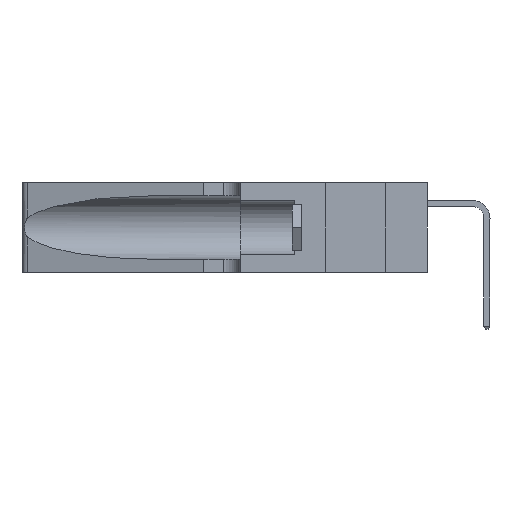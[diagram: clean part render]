
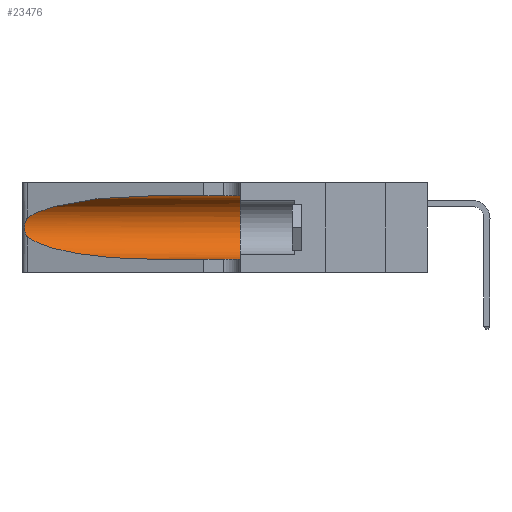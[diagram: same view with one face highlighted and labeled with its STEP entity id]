
A CAD part, left-side view. The second image highlights one B-rep face of the part: STEP entity #23476.
In plain terms, the highlighted cylindrical face has radius 3.308 mm (diameter 6.617 mm), a partial arc.
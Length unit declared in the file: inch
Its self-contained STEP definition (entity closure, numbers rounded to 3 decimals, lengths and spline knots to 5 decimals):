
#197 = VERTEX_POINT ( 'NONE', #7270 ) ;
#234 =( BOUNDED_CURVE ( )  B_SPLINE_CURVE ( 3, ( #10838, #6887, #12788, #996 ),
 .UNSPECIFIED., .F., .F. ) 
 B_SPLINE_CURVE_WITH_KNOTS ( ( 4, 4 ),
 ( 1.5708, 2.84003 ),
 .UNSPECIFIED. ) 
 CURVE ( )  GEOMETRIC_REPRESENTATION_ITEM ( )  RATIONAL_B_SPLINE_CURVE ( ( 1., 0.87, 0.87, 1. ) ) 
 REPRESENTATION_ITEM ( '' )  );
#996 = CARTESIAN_POINT ( 'NONE',  ( 0.25487, 1.22718, 0.22369 ) ) ;
#1383 = CARTESIAN_POINT ( 'NONE',  ( 0.1305, 0.72297, 0.05475 ) ) ;
#1867 = CARTESIAN_POINT ( 'NONE',  ( 0.25854, 1.2359, 0.20912 ) ) ;
#3170 = EDGE_CURVE ( 'NONE', #6573, #18868, #19099, .T. ) ;
#3399 = CARTESIAN_POINT ( 'NONE',  ( 0.1305, 0.35, 0.31525 ) ) ;
#3686 = VERTEX_POINT ( 'NONE', #19341 ) ;
#3841 = CARTESIAN_POINT ( 'NONE',  ( 0.26075, 1.23896, 0.19203 ) ) ;
#3850 = CARTESIAN_POINT ( 'NONE',  ( 0.1305, 1.61858, 0.05475 ) ) ;
#4931 = CIRCLE ( 'NONE', #16431, 0.13025 ) ;
#5679 = EDGE_CURVE ( 'NONE', #18096, #3686, #4931, .T. ) ;
#5727 = ORIENTED_EDGE ( 'NONE', *, *, #15641, .T. ) ;
#5842 = CARTESIAN_POINT ( 'NONE',  ( 0.26017, 1.23833, 0.17102 ) ) ;
#5984 = DIRECTION ( 'NONE',  ( 0., 0., -1. ) ) ;
#6308 = ORIENTED_EDGE ( 'NONE', *, *, #7146, .T. ) ;
#6573 = VERTEX_POINT ( 'NONE', #15564 ) ;
#6686 = AXIS2_PLACEMENT_3D ( 'NONE', #7915, #17740, #5984 ) ;
#6887 = CARTESIAN_POINT ( 'NONE',  ( 0.18966, 0.96281, 0.31525 ) ) ;
#7146 = EDGE_CURVE ( 'NONE', #9513, #6573, #13261, .T. ) ;
#7270 = CARTESIAN_POINT ( 'NONE',  ( 0.1305, 0.72297, 0.31525 ) ) ;
#7305 = ORIENTED_EDGE ( 'NONE', *, *, #3170, .T. ) ;
#7864 = CARTESIAN_POINT ( 'NONE',  ( 0.25789, 1.23486, 0.15765 ) ) ;
#7915 = CARTESIAN_POINT ( 'NONE',  ( 0.1305, 1.61858, 0.185 ) ) ;
#8028 = DIRECTION ( 'NONE',  ( 0., 1., 0. ) ) ;
#8555 = ORIENTED_EDGE ( 'NONE', *, *, #11719, .F. ) ;
#9513 = VERTEX_POINT ( 'NONE', #10595 ) ;
#9820 = CARTESIAN_POINT ( 'NONE',  ( 0.25555, 1.22993, 0.14849 ) ) ;
#10198 = CARTESIAN_POINT ( 'NONE',  ( 0.1305, 0.72297, 0.05475 ) ) ;
#10595 = CARTESIAN_POINT ( 'NONE',  ( 0.25487, 1.22718, 0.22369 ) ) ;
#10838 = CARTESIAN_POINT ( 'NONE',  ( 0.1305, 0.72297, 0.31525 ) ) ;
#11719 = EDGE_CURVE ( 'NONE', #197, #18096, #17333, .T. ) ;
#11855 = DIRECTION ( 'NONE',  ( 0., -1., 0. ) ) ;
#12130 = VECTOR ( 'NONE', #11855, 39.37008 ) ;
#12788 = CARTESIAN_POINT ( 'NONE',  ( 0.2373, 1.15595, 0.28018 ) ) ;
#13184 = CARTESIAN_POINT ( 'NONE',  ( 0.25487, 1.22718, 0.14631 ) ) ;
#13261 = B_SPLINE_CURVE_WITH_KNOTS ( 'NONE', 3,
 ( #23358, #21391, #25306, #13660, #1867, #15634, #3841, #17598, #5842, #19524, #7864, #21470, #9820, #23446 ),
 .UNSPECIFIED., .F., .F.,
 ( 4, 2, 2, 2, 2, 2, 4 ),
 ( 0., 0.00027, 0.00053, 0.00107, 0.0016, 0.00187, 0.00214 ),
 .UNSPECIFIED. ) ;
#13660 = CARTESIAN_POINT ( 'NONE',  ( 0.25787, 1.23484, 0.2124 ) ) ;
#13671 = DIRECTION ( 'NONE',  ( 0., -1., 0. ) ) ;
#13778 = LINE ( 'NONE', #3850, #18355 ) ;
#13823 = CARTESIAN_POINT ( 'NONE',  ( 0.1305, 1.61858, 0.31525 ) ) ;
#15351 = FACE_OUTER_BOUND ( 'NONE', #18845, .T. ) ;
#15564 = CARTESIAN_POINT ( 'NONE',  ( 0.25487, 1.22718, 0.14631 ) ) ;
#15634 = CARTESIAN_POINT ( 'NONE',  ( 0.26018, 1.23835, 0.19895 ) ) ;
#15641 = EDGE_CURVE ( 'NONE', #18868, #3686, #13778, .T. ) ;
#16431 = AXIS2_PLACEMENT_3D ( 'NONE', #19682, #8028, #21636 ) ;
#16506 = EDGE_CURVE ( 'NONE', #197, #9513, #234, .T. ) ;
#17333 = LINE ( 'NONE', #13823, #12130 ) ;
#17598 = CARTESIAN_POINT ( 'NONE',  ( 0.26075, 1.23896, 0.178 ) ) ;
#17740 = DIRECTION ( 'NONE',  ( 0., -1., 0. ) ) ;
#18096 = VERTEX_POINT ( 'NONE', #3399 ) ;
#18355 = VECTOR ( 'NONE', #13671, 39.37008 ) ;
#18845 = EDGE_LOOP ( 'NONE', ( #22791, #6308, #7305, #5727, #24990, #8555 ) ) ;
#18868 = VERTEX_POINT ( 'NONE', #10198 ) ;
#18883 = CARTESIAN_POINT ( 'NONE',  ( 0.18966, 0.96281, 0.05475 ) ) ;
#19099 =( BOUNDED_CURVE ( )  B_SPLINE_CURVE ( 3, ( #13184, #22871, #18883, #1383 ),
 .UNSPECIFIED., .F., .F. ) 
 B_SPLINE_CURVE_WITH_KNOTS ( ( 4, 4 ),
 ( 3.44316, 4.71239 ),
 .UNSPECIFIED. ) 
 CURVE ( )  GEOMETRIC_REPRESENTATION_ITEM ( )  RATIONAL_B_SPLINE_CURVE ( ( 1., 0.87, 0.87, 1. ) ) 
 REPRESENTATION_ITEM ( '' )  );
#19288 = CYLINDRICAL_SURFACE ( 'NONE', #6686, 0.13025 ) ;
#19341 = CARTESIAN_POINT ( 'NONE',  ( 0.1305, 0.35, 0.05475 ) ) ;
#19524 = CARTESIAN_POINT ( 'NONE',  ( 0.25856, 1.23593, 0.16098 ) ) ;
#19682 = CARTESIAN_POINT ( 'NONE',  ( 0.1305, 0.35, 0.185 ) ) ;
#21391 = CARTESIAN_POINT ( 'NONE',  ( 0.25555, 1.22994, 0.2215 ) ) ;
#21470 = CARTESIAN_POINT ( 'NONE',  ( 0.25639, 1.23186, 0.15144 ) ) ;
#21636 = DIRECTION ( 'NONE',  ( 0., 0., 1. ) ) ;
#22791 = ORIENTED_EDGE ( 'NONE', *, *, #16506, .T. ) ;
#22871 = CARTESIAN_POINT ( 'NONE',  ( 0.2373, 1.15595, 0.08982 ) ) ;
#23358 = CARTESIAN_POINT ( 'NONE',  ( 0.25487, 1.22718, 0.22369 ) ) ;
#23446 = CARTESIAN_POINT ( 'NONE',  ( 0.25487, 1.22718, 0.14631 ) ) ;
#23476 = ADVANCED_FACE ( 'NONE', ( #15351 ), #19288, .F. ) ;
#24990 = ORIENTED_EDGE ( 'NONE', *, *, #5679, .F. ) ;
#25306 = CARTESIAN_POINT ( 'NONE',  ( 0.25639, 1.23184, 0.21858 ) ) ;
